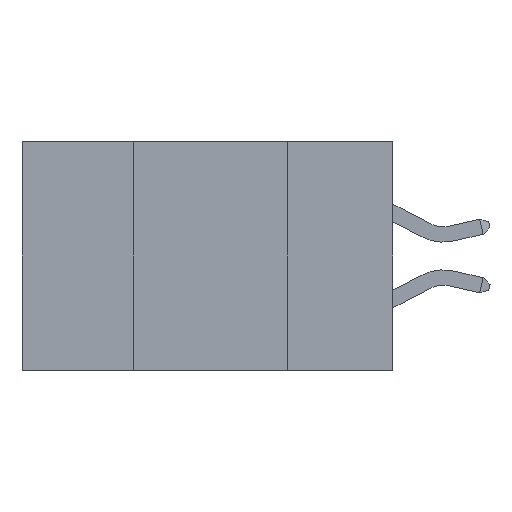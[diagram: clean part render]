
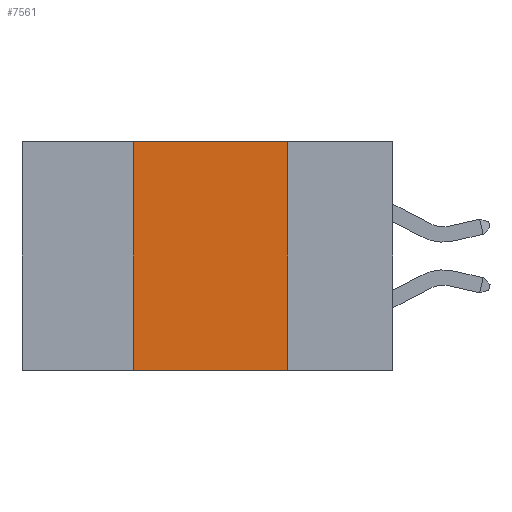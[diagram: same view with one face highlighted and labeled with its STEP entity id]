
A CAD part, left-side view. The second image highlights one B-rep face of the part: STEP entity #7561.
In plain terms, the highlighted planar face has unit normal (-1, 0, 0).
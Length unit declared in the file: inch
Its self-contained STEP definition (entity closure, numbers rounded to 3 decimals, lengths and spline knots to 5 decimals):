
#958 = EDGE_LOOP ( 'NONE', ( #21904, #15090, #9943, #1914 ) ) ;
#1549 = VECTOR ( 'NONE', #6753, 39.37008 ) ;
#1914 = ORIENTED_EDGE ( 'NONE', *, *, #18150, .T. ) ;
#2357 = EDGE_CURVE ( 'NONE', #17369, #7029, #18639, .T. ) ;
#2358 = PLANE ( 'NONE',  #13013 ) ;
#4134 = VECTOR ( 'NONE', #5694, 39.37008 ) ;
#4242 = DIRECTION ( 'NONE',  ( 1., 0., 0. ) ) ;
#5624 = DIRECTION ( 'NONE',  ( 0., 0., -1. ) ) ;
#5694 = DIRECTION ( 'NONE',  ( 0., -1., 0. ) ) ;
#6593 = EDGE_CURVE ( 'NONE', #6710, #21808, #16360, .T. ) ;
#6710 = VERTEX_POINT ( 'NONE', #20715 ) ;
#6753 = DIRECTION ( 'NONE',  ( 0., 0., 1. ) ) ;
#7029 = VERTEX_POINT ( 'NONE', #16621 ) ;
#7561 = ADVANCED_FACE ( 'NONE', ( #10407 ), #2358, .F. ) ;
#8420 = DIRECTION ( 'NONE',  ( 0., -1., 0. ) ) ;
#8477 = CARTESIAN_POINT ( 'NONE',  ( 0., 0.42, 0. ) ) ;
#9215 = CARTESIAN_POINT ( 'NONE',  ( 0., 0.17, 0. ) ) ;
#9943 = ORIENTED_EDGE ( 'NONE', *, *, #6593, .F. ) ;
#10407 = FACE_OUTER_BOUND ( 'NONE', #958, .T. ) ;
#10783 = CARTESIAN_POINT ( 'NONE',  ( 0., 0.42, 0. ) ) ;
#12958 = VECTOR ( 'NONE', #8420, 39.37008 ) ;
#13013 = AXIS2_PLACEMENT_3D ( 'NONE', #14873, #4242, #16592 ) ;
#14691 = EDGE_CURVE ( 'NONE', #21808, #17369, #18108, .T. ) ;
#14873 = CARTESIAN_POINT ( 'NONE',  ( 0., 0.6, 0. ) ) ;
#15090 = ORIENTED_EDGE ( 'NONE', *, *, #14691, .F. ) ;
#16360 = LINE ( 'NONE', #8477, #1549 ) ;
#16592 = DIRECTION ( 'NONE',  ( 0., 0., -1. ) ) ;
#16621 = CARTESIAN_POINT ( 'NONE',  ( 0., 0.17, -0.37 ) ) ;
#17024 = CARTESIAN_POINT ( 'NONE',  ( 0., 0.6, -0.37 ) ) ;
#17369 = VERTEX_POINT ( 'NONE', #20150 ) ;
#17905 = CARTESIAN_POINT ( 'NONE',  ( 0., 0.6, 0. ) ) ;
#18108 = LINE ( 'NONE', #17905, #4134 ) ;
#18128 = VECTOR ( 'NONE', #5624, 39.37008 ) ;
#18150 = EDGE_CURVE ( 'NONE', #6710, #7029, #18530, .T. ) ;
#18530 = LINE ( 'NONE', #17024, #12958 ) ;
#18639 = LINE ( 'NONE', #9215, #18128 ) ;
#20150 = CARTESIAN_POINT ( 'NONE',  ( 0., 0.17, 0. ) ) ;
#20715 = CARTESIAN_POINT ( 'NONE',  ( 0., 0.42, -0.37 ) ) ;
#21808 = VERTEX_POINT ( 'NONE', #10783 ) ;
#21904 = ORIENTED_EDGE ( 'NONE', *, *, #2357, .F. ) ;
